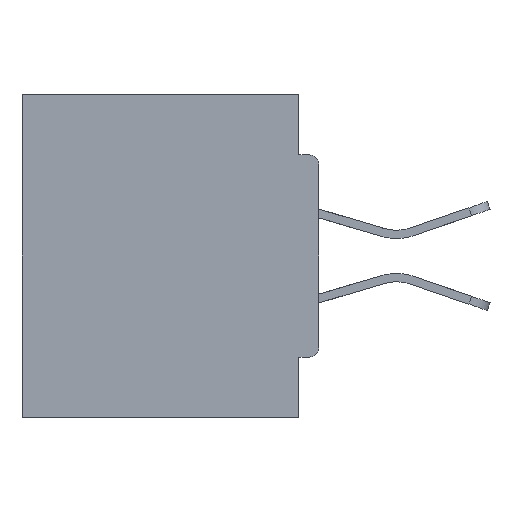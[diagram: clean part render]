
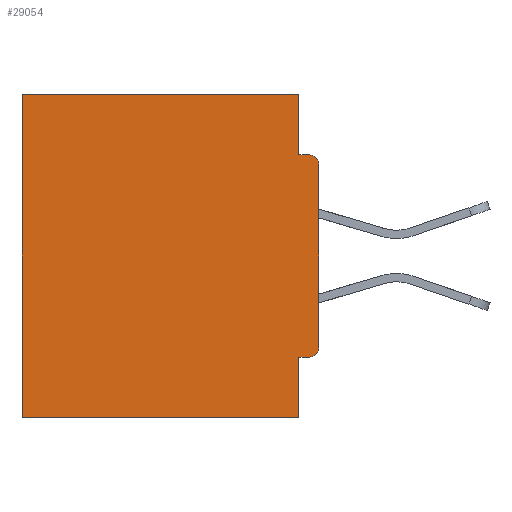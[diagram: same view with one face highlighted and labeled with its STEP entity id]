
A CAD part, left-side view. The second image highlights one B-rep face of the part: STEP entity #29054.
In plain terms, the highlighted planar face has unit normal (-1, 0, 0).
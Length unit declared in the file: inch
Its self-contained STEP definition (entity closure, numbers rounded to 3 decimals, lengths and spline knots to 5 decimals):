
#214 = DIRECTION ( 'NONE',  ( 0., 0., -1. ) ) ;
#222 = ORIENTED_EDGE ( 'NONE', *, *, #30499, .T. ) ;
#1338 = DIRECTION ( 'NONE',  ( 0., 0., -1. ) ) ;
#1479 = CARTESIAN_POINT ( 'NONE',  ( 0.298, 0.031, -0.5 ) ) ;
#1667 = AXIS2_PLACEMENT_3D ( 'NONE', #34501, #13081, #28994 ) ;
#1714 = CARTESIAN_POINT ( 'NONE',  ( 0.298, 0.031, -0.0935 ) ) ;
#2290 = VERTEX_POINT ( 'NONE', #19622 ) ;
#2349 = CARTESIAN_POINT ( 'NONE',  ( 0.298, 0., -0.0935 ) ) ;
#2920 = CARTESIAN_POINT ( 'NONE',  ( 0.298, 0., 0. ) ) ;
#3320 = DIRECTION ( 'NONE',  ( -1., 0., 0. ) ) ;
#3687 = ORIENTED_EDGE ( 'NONE', *, *, #24177, .F. ) ;
#5218 = DIRECTION ( 'NONE',  ( 0., -1., 0. ) ) ;
#5551 = DIRECTION ( 'NONE',  ( 0., 0., -1. ) ) ;
#5715 = LINE ( 'NONE', #24589, #26535 ) ;
#5780 = DIRECTION ( 'NONE',  ( 0., 0., -1. ) ) ;
#6698 = VECTOR ( 'NONE', #14094, 39.37008 ) ;
#7208 = CARTESIAN_POINT ( 'NONE',  ( 0.298, 0.015, -0.4065 ) ) ;
#7753 = VERTEX_POINT ( 'NONE', #24570 ) ;
#8255 = EDGE_CURVE ( 'NONE', #10827, #16009, #19720, .T. ) ;
#8471 = DIRECTION ( 'NONE',  ( 0., 0., -1. ) ) ;
#9455 = DIRECTION ( 'NONE',  ( 0., 1., 0. ) ) ;
#10109 = EDGE_CURVE ( 'NONE', #11049, #29907, #22133, .T. ) ;
#10170 = VECTOR ( 'NONE', #1338, 39.37008 ) ;
#10543 = CARTESIAN_POINT ( 'NONE',  ( 0.298, 0., -0.3915 ) ) ;
#10827 = VERTEX_POINT ( 'NONE', #1714 ) ;
#10865 = CARTESIAN_POINT ( 'NONE',  ( 0.298, 0., -0.1085 ) ) ;
#11026 = PLANE ( 'NONE',  #17103 ) ;
#11035 = EDGE_CURVE ( 'NONE', #31675, #33251, #13527, .T. ) ;
#11049 = VERTEX_POINT ( 'NONE', #10865 ) ;
#11431 = CARTESIAN_POINT ( 'NONE',  ( 0.298, 0.46, -0.5 ) ) ;
#11962 = CARTESIAN_POINT ( 'NONE',  ( 0.298, 0., -0.4065 ) ) ;
#12180 = CARTESIAN_POINT ( 'NONE',  ( 0.298, 0., 0. ) ) ;
#12923 = VECTOR ( 'NONE', #30987, 39.37008 ) ;
#13081 = DIRECTION ( 'NONE',  ( -1., 0., 0. ) ) ;
#13117 = EDGE_CURVE ( 'NONE', #25786, #33251, #5715, .T. ) ;
#13527 = LINE ( 'NONE', #27500, #6698 ) ;
#13990 = EDGE_CURVE ( 'NONE', #17323, #29907, #25653, .T. ) ;
#14094 = DIRECTION ( 'NONE',  ( 0., 1., 0. ) ) ;
#14137 = LINE ( 'NONE', #14440, #22641 ) ;
#14440 = CARTESIAN_POINT ( 'NONE',  ( 0.298, 0., 0. ) ) ;
#14707 = LINE ( 'NONE', #11962, #15985 ) ;
#15123 = CARTESIAN_POINT ( 'NONE',  ( 0.298, 0.46, 0. ) ) ;
#15985 = VECTOR ( 'NONE', #9455, 39.37008 ) ;
#16009 = VERTEX_POINT ( 'NONE', #29696 ) ;
#16835 = ORIENTED_EDGE ( 'NONE', *, *, #28990, .F. ) ;
#17103 = AXIS2_PLACEMENT_3D ( 'NONE', #2920, #27769, #5551 ) ;
#17227 = EDGE_LOOP ( 'NONE', ( #29567, #27878, #16835, #222, #27812, #33244, #3687, #22797, #28729, #34397 ) ) ;
#17323 = VERTEX_POINT ( 'NONE', #7208 ) ;
#19397 = LINE ( 'NONE', #27423, #32105 ) ;
#19622 = CARTESIAN_POINT ( 'NONE',  ( 0.298, 0.031, 0. ) ) ;
#19720 = LINE ( 'NONE', #2349, #32032 ) ;
#19793 = LINE ( 'NONE', #1479, #12923 ) ;
#22133 = LINE ( 'NONE', #12180, #10170 ) ;
#22641 = VECTOR ( 'NONE', #27504, 39.37008 ) ;
#22797 = ORIENTED_EDGE ( 'NONE', *, *, #28603, .F. ) ;
#23138 = AXIS2_PLACEMENT_3D ( 'NONE', #30433, #3320, #8471 ) ;
#24177 = EDGE_CURVE ( 'NONE', #7753, #31675, #19793, .T. ) ;
#24570 = CARTESIAN_POINT ( 'NONE',  ( 0.298, 0.031, -0.4065 ) ) ;
#24589 = CARTESIAN_POINT ( 'NONE',  ( 0.298, 0.46, 0. ) ) ;
#25653 = CIRCLE ( 'NONE', #23138, 0.015 ) ;
#25786 = VERTEX_POINT ( 'NONE', #15123 ) ;
#26535 = VECTOR ( 'NONE', #214, 39.37008 ) ;
#27190 = CARTESIAN_POINT ( 'NONE',  ( 0.298, 0.031, -0.5 ) ) ;
#27423 = CARTESIAN_POINT ( 'NONE',  ( 0.298, 0.031, -0.5 ) ) ;
#27500 = CARTESIAN_POINT ( 'NONE',  ( 0.298, 0., -0.5 ) ) ;
#27504 = DIRECTION ( 'NONE',  ( 0., 1., 0. ) ) ;
#27769 = DIRECTION ( 'NONE',  ( 1., 0., 0. ) ) ;
#27812 = ORIENTED_EDGE ( 'NONE', *, *, #13117, .T. ) ;
#27878 = ORIENTED_EDGE ( 'NONE', *, *, #8255, .F. ) ;
#28603 = EDGE_CURVE ( 'NONE', #17323, #7753, #14707, .T. ) ;
#28729 = ORIENTED_EDGE ( 'NONE', *, *, #13990, .T. ) ;
#28990 = EDGE_CURVE ( 'NONE', #2290, #10827, #19397, .T. ) ;
#28994 = DIRECTION ( 'NONE',  ( 0., 0., -1. ) ) ;
#29054 = ADVANCED_FACE ( 'NONE', ( #30810 ), #11026, .F. ) ;
#29380 = CIRCLE ( 'NONE', #1667, 0.015 ) ;
#29567 = ORIENTED_EDGE ( 'NONE', *, *, #34669, .T. ) ;
#29696 = CARTESIAN_POINT ( 'NONE',  ( 0.298, 0.015, -0.0935 ) ) ;
#29907 = VERTEX_POINT ( 'NONE', #10543 ) ;
#30433 = CARTESIAN_POINT ( 'NONE',  ( 0.298, 0.015, -0.3915 ) ) ;
#30499 = EDGE_CURVE ( 'NONE', #2290, #25786, #14137, .T. ) ;
#30810 = FACE_OUTER_BOUND ( 'NONE', #17227, .T. ) ;
#30987 = DIRECTION ( 'NONE',  ( 0., 0., -1. ) ) ;
#31675 = VERTEX_POINT ( 'NONE', #27190 ) ;
#32032 = VECTOR ( 'NONE', #5218, 39.37008 ) ;
#32105 = VECTOR ( 'NONE', #5780, 39.37008 ) ;
#33244 = ORIENTED_EDGE ( 'NONE', *, *, #11035, .F. ) ;
#33251 = VERTEX_POINT ( 'NONE', #11431 ) ;
#34397 = ORIENTED_EDGE ( 'NONE', *, *, #10109, .F. ) ;
#34501 = CARTESIAN_POINT ( 'NONE',  ( 0.298, 0.015, -0.1085 ) ) ;
#34669 = EDGE_CURVE ( 'NONE', #11049, #16009, #29380, .T. ) ;
